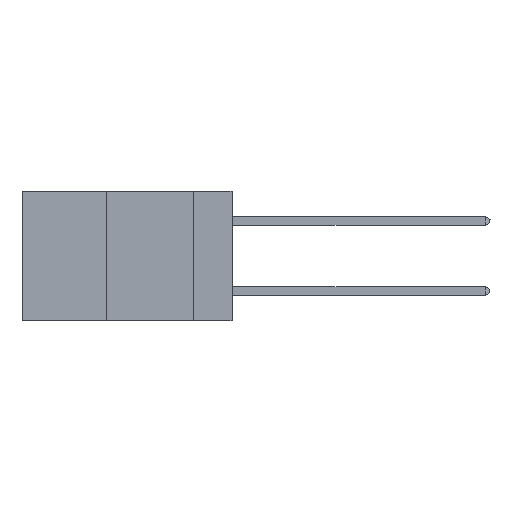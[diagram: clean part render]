
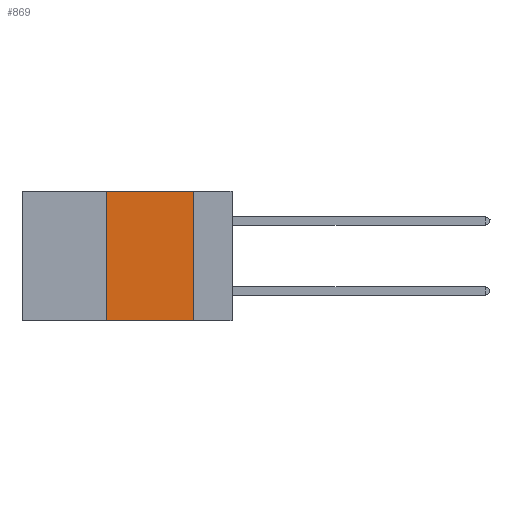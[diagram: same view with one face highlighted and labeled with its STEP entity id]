
A CAD part, left-side view. The second image highlights one B-rep face of the part: STEP entity #869.
In plain terms, the highlighted planar face has unit normal (-1, 0, 0).
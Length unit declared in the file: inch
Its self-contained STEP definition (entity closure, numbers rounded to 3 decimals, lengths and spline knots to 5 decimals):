
#187 = VERTEX_POINT ( 'NONE', #9506 ) ;
#454 = PLANE ( 'NONE',  #11218 ) ;
#869 = ADVANCED_FACE ( 'NONE', ( #9606 ), #454, .F. ) ;
#1132 = ORIENTED_EDGE ( 'NONE', *, *, #11763, .F. ) ;
#1475 = LINE ( 'NONE', #5620, #3498 ) ;
#2556 = DIRECTION ( 'NONE',  ( 0., -1., 0. ) ) ;
#3202 = ORIENTED_EDGE ( 'NONE', *, *, #4742, .T. ) ;
#3493 = CARTESIAN_POINT ( 'NONE',  ( 0., 0.36, 0. ) ) ;
#3498 = VECTOR ( 'NONE', #5680, 39.37008 ) ;
#3534 = DIRECTION ( 'NONE',  ( 1., 0., 0. ) ) ;
#3622 = ORIENTED_EDGE ( 'NONE', *, *, #10582, .F. ) ;
#3759 = CARTESIAN_POINT ( 'NONE',  ( 0., 0.36, -0.37 ) ) ;
#4048 = VECTOR ( 'NONE', #8834, 39.37008 ) ;
#4424 = LINE ( 'NONE', #8755, #6357 ) ;
#4533 = CARTESIAN_POINT ( 'NONE',  ( 0., 0.6, 0. ) ) ;
#4742 = EDGE_CURVE ( 'NONE', #6231, #9605, #1475, .T. ) ;
#4789 = EDGE_CURVE ( 'NONE', #6231, #187, #7594, .T. ) ;
#5375 = VERTEX_POINT ( 'NONE', #7077 ) ;
#5620 = CARTESIAN_POINT ( 'NONE',  ( 0., 0.6, -0.37 ) ) ;
#5680 = DIRECTION ( 'NONE',  ( 0., -1., 0. ) ) ;
#5802 = CARTESIAN_POINT ( 'NONE',  ( 0., 0.11, -0.37 ) ) ;
#6231 = VERTEX_POINT ( 'NONE', #3759 ) ;
#6357 = VECTOR ( 'NONE', #2556, 39.37008 ) ;
#6606 = CARTESIAN_POINT ( 'NONE',  ( 0., 0.11, 0. ) ) ;
#7077 = CARTESIAN_POINT ( 'NONE',  ( 0., 0.11, 0. ) ) ;
#7574 = DIRECTION ( 'NONE',  ( 0., 0., -1. ) ) ;
#7594 = LINE ( 'NONE', #3493, #8823 ) ;
#8325 = ORIENTED_EDGE ( 'NONE', *, *, #4789, .F. ) ;
#8559 = DIRECTION ( 'NONE',  ( 0., 0., 1. ) ) ;
#8755 = CARTESIAN_POINT ( 'NONE',  ( 0., 0.6, 0. ) ) ;
#8766 = LINE ( 'NONE', #6606, #4048 ) ;
#8823 = VECTOR ( 'NONE', #8559, 39.37008 ) ;
#8834 = DIRECTION ( 'NONE',  ( 0., 0., -1. ) ) ;
#9359 = EDGE_LOOP ( 'NONE', ( #1132, #3622, #8325, #3202 ) ) ;
#9506 = CARTESIAN_POINT ( 'NONE',  ( 0., 0.36, 0. ) ) ;
#9605 = VERTEX_POINT ( 'NONE', #5802 ) ;
#9606 = FACE_OUTER_BOUND ( 'NONE', #9359, .T. ) ;
#10582 = EDGE_CURVE ( 'NONE', #187, #5375, #4424, .T. ) ;
#11218 = AXIS2_PLACEMENT_3D ( 'NONE', #4533, #3534, #7574 ) ;
#11763 = EDGE_CURVE ( 'NONE', #5375, #9605, #8766, .T. ) ;
